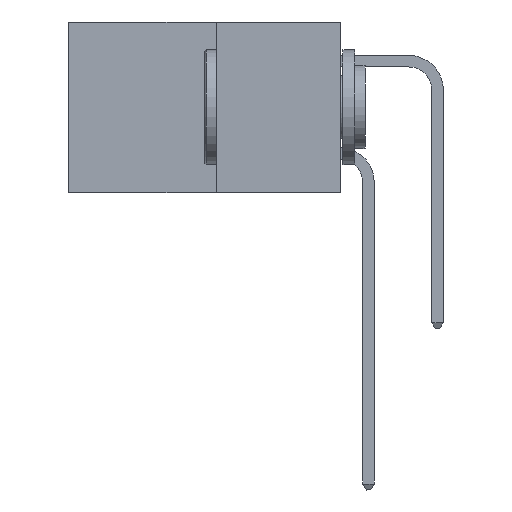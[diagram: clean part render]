
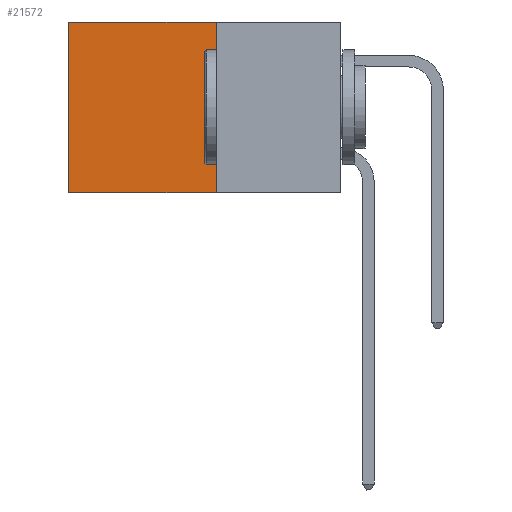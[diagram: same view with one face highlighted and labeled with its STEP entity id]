
A CAD part, left-side view. The second image highlights one B-rep face of the part: STEP entity #21572.
In plain terms, the highlighted planar face has unit normal (-1, 0, 0).
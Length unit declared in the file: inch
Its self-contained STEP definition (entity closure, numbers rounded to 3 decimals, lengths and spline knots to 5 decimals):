
#50 = LINE ( 'NONE', #15905, #9184 ) ;
#335 = PLANE ( 'NONE',  #6940 ) ;
#799 = ORIENTED_EDGE ( 'NONE', *, *, #20011, .F. ) ;
#1065 = ORIENTED_EDGE ( 'NONE', *, *, #20416, .F. ) ;
#1105 = CARTESIAN_POINT ( 'NONE',  ( 0.277, 0.27, 0. ) ) ;
#2850 = EDGE_CURVE ( 'NONE', #10662, #21932, #16908, .T. ) ;
#2921 = ORIENTED_EDGE ( 'NONE', *, *, #18108, .T. ) ;
#3487 = VERTEX_POINT ( 'NONE', #4023 ) ;
#4023 = CARTESIAN_POINT ( 'NONE',  ( 0.277, 0.27, -0.37 ) ) ;
#5831 = CARTESIAN_POINT ( 'NONE',  ( 0.277, 0.27, -0.37 ) ) ;
#6000 = DIRECTION ( 'NONE',  ( 0., 0., -1. ) ) ;
#6428 = FACE_OUTER_BOUND ( 'NONE', #21792, .T. ) ;
#6487 = CARTESIAN_POINT ( 'NONE',  ( 0.277, 0.59, 0. ) ) ;
#6917 = CARTESIAN_POINT ( 'NONE',  ( 0.277, 0.59, -0.37 ) ) ;
#6940 = AXIS2_PLACEMENT_3D ( 'NONE', #5831, #9490, #21897 ) ;
#7303 = VECTOR ( 'NONE', #6000, 39.37008 ) ;
#8475 = LINE ( 'NONE', #22388, #21576 ) ;
#8591 = CARTESIAN_POINT ( 'NONE',  ( 0.277, 0.27, -0.37 ) ) ;
#8719 = DIRECTION ( 'NONE',  ( 0., 1., 0. ) ) ;
#9184 = VECTOR ( 'NONE', #8719, 39.37008 ) ;
#9490 = DIRECTION ( 'NONE',  ( 1., 0., 0. ) ) ;
#9498 = VERTEX_POINT ( 'NONE', #1105 ) ;
#10405 = DIRECTION ( 'NONE',  ( 0., 0., -1. ) ) ;
#10662 = VERTEX_POINT ( 'NONE', #6487 ) ;
#10724 = CARTESIAN_POINT ( 'NONE',  ( 0.277, 0.59, -0.37 ) ) ;
#11841 = DIRECTION ( 'NONE',  ( 0., 1., 0. ) ) ;
#12216 = LINE ( 'NONE', #8591, #21034 ) ;
#15905 = CARTESIAN_POINT ( 'NONE',  ( 0.277, 0.27, 0. ) ) ;
#16802 = ORIENTED_EDGE ( 'NONE', *, *, #2850, .T. ) ;
#16908 = LINE ( 'NONE', #10724, #7303 ) ;
#18108 = EDGE_CURVE ( 'NONE', #9498, #10662, #50, .T. ) ;
#20011 = EDGE_CURVE ( 'NONE', #9498, #3487, #12216, .T. ) ;
#20416 = EDGE_CURVE ( 'NONE', #3487, #21932, #8475, .T. ) ;
#21034 = VECTOR ( 'NONE', #10405, 39.37008 ) ;
#21572 = ADVANCED_FACE ( 'NONE', ( #6428 ), #335, .F. ) ;
#21576 = VECTOR ( 'NONE', #11841, 39.37008 ) ;
#21792 = EDGE_LOOP ( 'NONE', ( #16802, #1065, #799, #2921 ) ) ;
#21897 = DIRECTION ( 'NONE',  ( 0., 0., -1. ) ) ;
#21932 = VERTEX_POINT ( 'NONE', #6917 ) ;
#22388 = CARTESIAN_POINT ( 'NONE',  ( 0.277, 0.27, -0.37 ) ) ;
